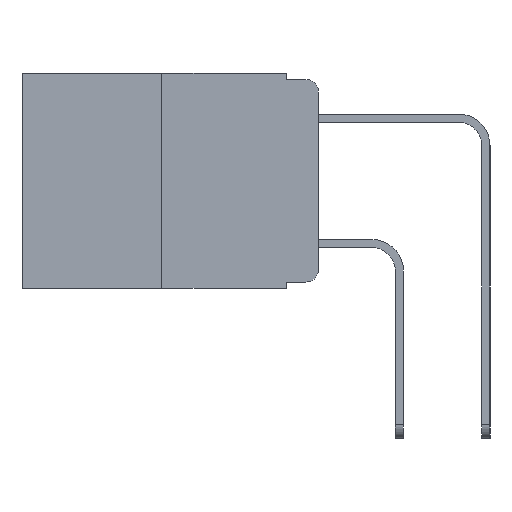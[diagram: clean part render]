
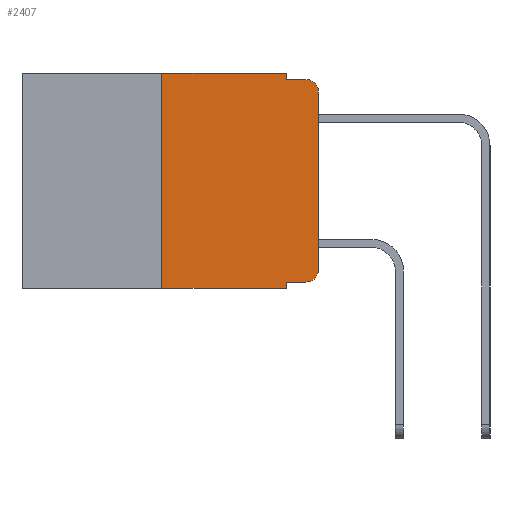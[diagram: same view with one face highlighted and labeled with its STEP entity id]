
A CAD part, left-side view. The second image highlights one B-rep face of the part: STEP entity #2407.
In plain terms, the highlighted planar face has unit normal (-1, 0, 0).
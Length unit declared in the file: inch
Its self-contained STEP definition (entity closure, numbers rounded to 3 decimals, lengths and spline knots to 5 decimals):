
#184 = ORIENTED_EDGE ( 'NONE', *, *, #6223, .T. ) ;
#461 = CARTESIAN_POINT ( 'NONE',  ( 0., 0.25, -0.343 ) ) ;
#567 = LINE ( 'NONE', #2111, #6657 ) ;
#582 = ORIENTED_EDGE ( 'NONE', *, *, #2688, .F. ) ;
#1171 = VECTOR ( 'NONE', #13158, 39.37008 ) ;
#1267 = EDGE_CURVE ( 'NONE', #14545, #15879, #2964, .T. ) ;
#1504 = DIRECTION ( 'NONE',  ( 0., 0., 1. ) ) ;
#1509 = VECTOR ( 'NONE', #2020, 39.37008 ) ;
#1554 = CARTESIAN_POINT ( 'NONE',  ( 0., 0., 0. ) ) ;
#1884 = CARTESIAN_POINT ( 'NONE',  ( 0., 0.473, 0. ) ) ;
#1926 = VECTOR ( 'NONE', #8448, 39.37008 ) ;
#1995 = CARTESIAN_POINT ( 'NONE',  ( 0., 0.051, -0.343 ) ) ;
#2020 = DIRECTION ( 'NONE',  ( 0., 0., -1. ) ) ;
#2111 = CARTESIAN_POINT ( 'NONE',  ( 0., 0.051, -0.333 ) ) ;
#2397 = ORIENTED_EDGE ( 'NONE', *, *, #13094, .T. ) ;
#2407 = ADVANCED_FACE ( 'NONE', ( #16250 ), #12792, .F. ) ;
#2688 = EDGE_CURVE ( 'NONE', #4084, #13371, #11856, .T. ) ;
#2816 = DIRECTION ( 'NONE',  ( -1., 0., 0. ) ) ;
#2964 = CIRCLE ( 'NONE', #8397, 0.02 ) ;
#3459 = DIRECTION ( 'NONE',  ( 0., 0., 1. ) ) ;
#3790 = DIRECTION ( 'NONE',  ( 0., 0., -1. ) ) ;
#4084 = VERTEX_POINT ( 'NONE', #7272 ) ;
#4129 = CARTESIAN_POINT ( 'NONE',  ( 0., 0.051, -0.01 ) ) ;
#4342 = VERTEX_POINT ( 'NONE', #11598 ) ;
#4458 = ORIENTED_EDGE ( 'NONE', *, *, #10833, .T. ) ;
#4502 = AXIS2_PLACEMENT_3D ( 'NONE', #5096, #6368, #15360 ) ;
#4666 = LINE ( 'NONE', #4129, #1171 ) ;
#4716 = DIRECTION ( 'NONE',  ( 0., -1., 0. ) ) ;
#5096 = CARTESIAN_POINT ( 'NONE',  ( 0., 0.473, 0. ) ) ;
#5347 = EDGE_CURVE ( 'NONE', #5798, #8554, #13360, .T. ) ;
#5602 = LINE ( 'NONE', #11538, #6006 ) ;
#5798 = VERTEX_POINT ( 'NONE', #461 ) ;
#6006 = VECTOR ( 'NONE', #3790, 39.37008 ) ;
#6194 = EDGE_CURVE ( 'NONE', #11710, #7420, #5602, .T. ) ;
#6223 = EDGE_CURVE ( 'NONE', #5798, #13371, #12043, .T. ) ;
#6275 = ORIENTED_EDGE ( 'NONE', *, *, #10526, .F. ) ;
#6368 = DIRECTION ( 'NONE',  ( 1., 0., 0. ) ) ;
#6506 = VECTOR ( 'NONE', #3459, 39.37008 ) ;
#6621 = CARTESIAN_POINT ( 'NONE',  ( 0., 0.02, -0.03 ) ) ;
#6657 = VECTOR ( 'NONE', #4716, 39.37008 ) ;
#6669 = ORIENTED_EDGE ( 'NONE', *, *, #5347, .F. ) ;
#7211 = CARTESIAN_POINT ( 'NONE',  ( 0., 0.02, -0.333 ) ) ;
#7272 = CARTESIAN_POINT ( 'NONE',  ( 0., 0.051, -0.333 ) ) ;
#7420 = VERTEX_POINT ( 'NONE', #9138 ) ;
#7943 = DIRECTION ( 'NONE',  ( 0., 0., -1. ) ) ;
#8261 = LINE ( 'NONE', #1554, #14677 ) ;
#8397 = AXIS2_PLACEMENT_3D ( 'NONE', #10596, #2816, #11884 ) ;
#8448 = DIRECTION ( 'NONE',  ( 0., -1., 0. ) ) ;
#8554 = VERTEX_POINT ( 'NONE', #10158 ) ;
#8782 = VERTEX_POINT ( 'NONE', #10656 ) ;
#9138 = CARTESIAN_POINT ( 'NONE',  ( 0., 0.051, -0.01 ) ) ;
#9613 = AXIS2_PLACEMENT_3D ( 'NONE', #6621, #15624, #7943 ) ;
#9764 = CIRCLE ( 'NONE', #9613, 0.02 ) ;
#9822 = CARTESIAN_POINT ( 'NONE',  ( 0., 0.051, 0. ) ) ;
#10158 = CARTESIAN_POINT ( 'NONE',  ( 0., 0.25, 0. ) ) ;
#10326 = CARTESIAN_POINT ( 'NONE',  ( 0., 0.473, -0.343 ) ) ;
#10526 = EDGE_CURVE ( 'NONE', #7420, #8782, #4666, .T. ) ;
#10596 = CARTESIAN_POINT ( 'NONE',  ( 0., 0.02, -0.313 ) ) ;
#10656 = CARTESIAN_POINT ( 'NONE',  ( 0., 0.02, -0.01 ) ) ;
#10833 = EDGE_CURVE ( 'NONE', #4084, #14545, #567, .T. ) ;
#11538 = CARTESIAN_POINT ( 'NONE',  ( 0., 0.051, 0. ) ) ;
#11598 = CARTESIAN_POINT ( 'NONE',  ( 0., 0., -0.03 ) ) ;
#11633 = VECTOR ( 'NONE', #16667, 39.37008 ) ;
#11710 = VERTEX_POINT ( 'NONE', #13132 ) ;
#11856 = LINE ( 'NONE', #9822, #1509 ) ;
#11884 = DIRECTION ( 'NONE',  ( 0., 0., -1. ) ) ;
#12043 = LINE ( 'NONE', #10326, #11633 ) ;
#12267 = LINE ( 'NONE', #1884, #1926 ) ;
#12792 = PLANE ( 'NONE',  #4502 ) ;
#13094 = EDGE_CURVE ( 'NONE', #4342, #8782, #9764, .T. ) ;
#13129 = ORIENTED_EDGE ( 'NONE', *, *, #6194, .F. ) ;
#13132 = CARTESIAN_POINT ( 'NONE',  ( 0., 0.051, 0. ) ) ;
#13158 = DIRECTION ( 'NONE',  ( 0., -1., 0. ) ) ;
#13360 = LINE ( 'NONE', #16312, #6506 ) ;
#13371 = VERTEX_POINT ( 'NONE', #1995 ) ;
#14149 = EDGE_LOOP ( 'NONE', ( #15724, #2397, #6275, #13129, #16501, #6669, #184, #582, #4458, #14726 ) ) ;
#14545 = VERTEX_POINT ( 'NONE', #7211 ) ;
#14677 = VECTOR ( 'NONE', #1504, 39.37008 ) ;
#14726 = ORIENTED_EDGE ( 'NONE', *, *, #1267, .T. ) ;
#15360 = DIRECTION ( 'NONE',  ( 0., 0., -1. ) ) ;
#15624 = DIRECTION ( 'NONE',  ( -1., 0., 0. ) ) ;
#15677 = EDGE_CURVE ( 'NONE', #15879, #4342, #8261, .T. ) ;
#15724 = ORIENTED_EDGE ( 'NONE', *, *, #15677, .T. ) ;
#15841 = EDGE_CURVE ( 'NONE', #8554, #11710, #12267, .T. ) ;
#15879 = VERTEX_POINT ( 'NONE', #16159 ) ;
#16159 = CARTESIAN_POINT ( 'NONE',  ( 0., 0., -0.313 ) ) ;
#16250 = FACE_OUTER_BOUND ( 'NONE', #14149, .T. ) ;
#16312 = CARTESIAN_POINT ( 'NONE',  ( 0., 0.25, 0. ) ) ;
#16501 = ORIENTED_EDGE ( 'NONE', *, *, #15841, .F. ) ;
#16667 = DIRECTION ( 'NONE',  ( 0., -1., 0. ) ) ;
